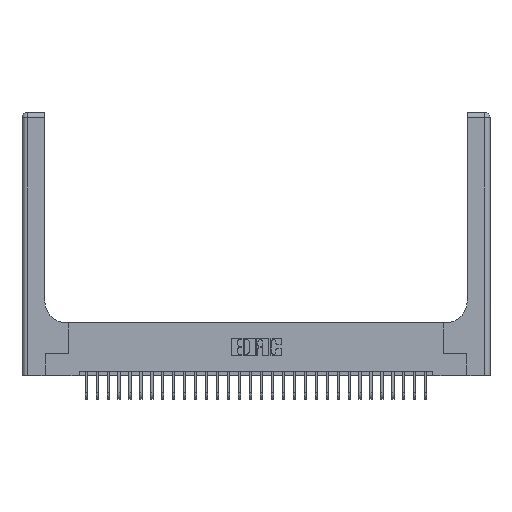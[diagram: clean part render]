
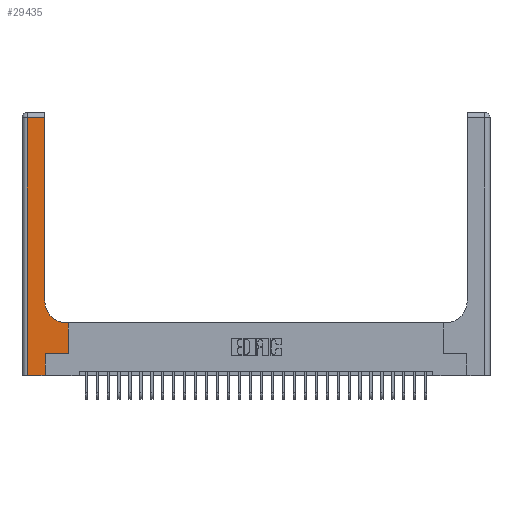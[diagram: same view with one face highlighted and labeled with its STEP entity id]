
A CAD part, top view. The second image highlights one B-rep face of the part: STEP entity #29435.
In plain terms, the highlighted planar face has unit normal (0, 0, 1).
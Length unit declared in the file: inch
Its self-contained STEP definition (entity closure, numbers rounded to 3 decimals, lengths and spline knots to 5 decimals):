
#43 = DIRECTION ( 'NONE',  ( 0., 0., -1. ) ) ;
#416 = VECTOR ( 'NONE', #1381, 39.37008 ) ;
#1381 = DIRECTION ( 'NONE',  ( 0., 1., 0. ) ) ;
#1811 = EDGE_CURVE ( 'NONE', #13115, #23577, #4561, .T. ) ;
#1951 = AXIS2_PLACEMENT_3D ( 'NONE', #4839, #43, #13989 ) ;
#2383 = EDGE_CURVE ( 'NONE', #8522, #23740, #24398, .T. ) ;
#2715 = CARTESIAN_POINT ( 'NONE',  ( 0.51, 0.85, 0.37 ) ) ;
#3863 = DIRECTION ( 'NONE',  ( -1., 0., 0. ) ) ;
#4275 = EDGE_CURVE ( 'NONE', #23029, #8522, #29350, .T. ) ;
#4489 = EDGE_CURVE ( 'NONE', #23577, #23029, #23021, .T. ) ;
#4561 = CIRCLE ( 'NONE', #5994, 0.25 ) ;
#4839 = CARTESIAN_POINT ( 'NONE',  ( 0., 3., 0.37 ) ) ;
#5113 = DIRECTION ( 'NONE',  ( 1., 0., 0. ) ) ;
#5994 = AXIS2_PLACEMENT_3D ( 'NONE', #2715, #7663, #5113 ) ;
#6059 = CARTESIAN_POINT ( 'NONE',  ( 0.26, 0.85, 0.37 ) ) ;
#7663 = DIRECTION ( 'NONE',  ( 0., 0., -1. ) ) ;
#8232 = ORIENTED_EDGE ( 'NONE', *, *, #4275, .T. ) ;
#8522 = VERTEX_POINT ( 'NONE', #9453 ) ;
#8781 = CARTESIAN_POINT ( 'NONE',  ( 0., 2.94, 0.37 ) ) ;
#9453 = CARTESIAN_POINT ( 'NONE',  ( 0.06, 2.94, 0.37 ) ) ;
#9552 = EDGE_CURVE ( 'NONE', #13191, #25147, #22629, .T. ) ;
#9608 = CARTESIAN_POINT ( 'NONE',  ( 0.528, 0.6, 0.37 ) ) ;
#9769 = CARTESIAN_POINT ( 'NONE',  ( 0., 0., 0.37 ) ) ;
#11032 = ORIENTED_EDGE ( 'NONE', *, *, #22211, .T. ) ;
#11645 = CARTESIAN_POINT ( 'NONE',  ( 0.26, 3., 0.37 ) ) ;
#12533 = ORIENTED_EDGE ( 'NONE', *, *, #4489, .T. ) ;
#12744 = ORIENTED_EDGE ( 'NONE', *, *, #26779, .T. ) ;
#13115 = VERTEX_POINT ( 'NONE', #16414 ) ;
#13191 = VERTEX_POINT ( 'NONE', #17016 ) ;
#13234 = DIRECTION ( 'NONE',  ( 0., 1., 0. ) ) ;
#13717 = VERTEX_POINT ( 'NONE', #9608 ) ;
#13873 = CARTESIAN_POINT ( 'NONE',  ( 0.26, 2.94, 0.37 ) ) ;
#13989 = DIRECTION ( 'NONE',  ( -1., 0., 0. ) ) ;
#14290 = LINE ( 'NONE', #9769, #22644 ) ;
#14928 = EDGE_LOOP ( 'NONE', ( #12533, #8232, #20110, #12744, #19065, #21750, #21232, #11032, #15663 ) ) ;
#15050 = CARTESIAN_POINT ( 'NONE',  ( 0.528, 0.25, 0.37 ) ) ;
#15663 = ORIENTED_EDGE ( 'NONE', *, *, #1811, .T. ) ;
#15921 = DIRECTION ( 'NONE',  ( 1., 0., 0. ) ) ;
#16414 = CARTESIAN_POINT ( 'NONE',  ( 0.51, 0.6, 0.37 ) ) ;
#17016 = CARTESIAN_POINT ( 'NONE',  ( 0.265, 0.25, 0.37 ) ) ;
#17182 = LINE ( 'NONE', #21772, #416 ) ;
#18331 = LINE ( 'NONE', #27319, #20764 ) ;
#19065 = ORIENTED_EDGE ( 'NONE', *, *, #26630, .T. ) ;
#20076 = EDGE_CURVE ( 'NONE', #25147, #13717, #17182, .T. ) ;
#20110 = ORIENTED_EDGE ( 'NONE', *, *, #2383, .T. ) ;
#20561 = CARTESIAN_POINT ( 'NONE',  ( 0.265, 0.25, 0.37 ) ) ;
#20764 = VECTOR ( 'NONE', #13234, 39.37008 ) ;
#20789 = DIRECTION ( 'NONE',  ( 0., 1., 0. ) ) ;
#20912 = VECTOR ( 'NONE', #20789, 39.37008 ) ;
#21098 = CARTESIAN_POINT ( 'NONE',  ( 0.265, 0., 0.37 ) ) ;
#21232 = ORIENTED_EDGE ( 'NONE', *, *, #20076, .T. ) ;
#21366 = VECTOR ( 'NONE', #27242, 39.37008 ) ;
#21750 = ORIENTED_EDGE ( 'NONE', *, *, #9552, .T. ) ;
#21772 = CARTESIAN_POINT ( 'NONE',  ( 0.528, 0.25, 0.37 ) ) ;
#21850 = LINE ( 'NONE', #26073, #24620 ) ;
#22211 = EDGE_CURVE ( 'NONE', #13717, #13115, #21850, .T. ) ;
#22231 = CARTESIAN_POINT ( 'NONE',  ( 0.06, 0., 0.37 ) ) ;
#22629 = LINE ( 'NONE', #20561, #26775 ) ;
#22644 = VECTOR ( 'NONE', #23551, 39.37008 ) ;
#23021 = LINE ( 'NONE', #11645, #20912 ) ;
#23029 = VERTEX_POINT ( 'NONE', #13873 ) ;
#23189 = VECTOR ( 'NONE', #26213, 39.37008 ) ;
#23551 = DIRECTION ( 'NONE',  ( 1., 0., 0. ) ) ;
#23577 = VERTEX_POINT ( 'NONE', #6059 ) ;
#23740 = VERTEX_POINT ( 'NONE', #22231 ) ;
#24398 = LINE ( 'NONE', #28480, #23189 ) ;
#24620 = VECTOR ( 'NONE', #3863, 39.37008 ) ;
#25147 = VERTEX_POINT ( 'NONE', #15050 ) ;
#25377 = PLANE ( 'NONE',  #1951 ) ;
#26073 = CARTESIAN_POINT ( 'NONE',  ( 0.26, 0.6, 0.37 ) ) ;
#26213 = DIRECTION ( 'NONE',  ( 0., -1., 0. ) ) ;
#26630 = EDGE_CURVE ( 'NONE', #27262, #13191, #18331, .T. ) ;
#26775 = VECTOR ( 'NONE', #15921, 39.37008 ) ;
#26779 = EDGE_CURVE ( 'NONE', #23740, #27262, #14290, .T. ) ;
#27191 = FACE_OUTER_BOUND ( 'NONE', #14928, .T. ) ;
#27242 = DIRECTION ( 'NONE',  ( -1., 0., 0. ) ) ;
#27262 = VERTEX_POINT ( 'NONE', #21098 ) ;
#27319 = CARTESIAN_POINT ( 'NONE',  ( 0.265, 0., 0.37 ) ) ;
#28480 = CARTESIAN_POINT ( 'NONE',  ( 0.06, 3., 0.37 ) ) ;
#29350 = LINE ( 'NONE', #8781, #21366 ) ;
#29435 = ADVANCED_FACE ( 'NONE', ( #27191 ), #25377, .F. ) ;
